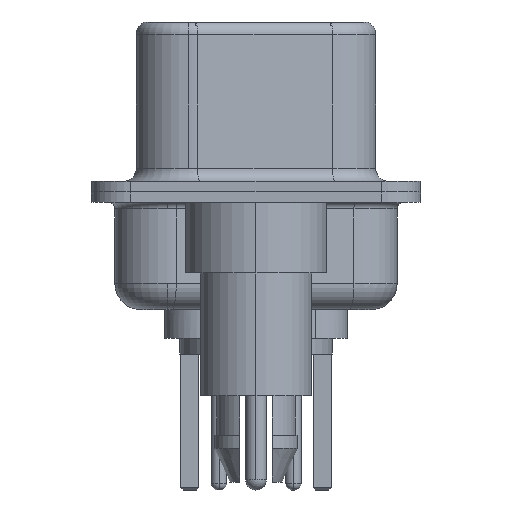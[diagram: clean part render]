
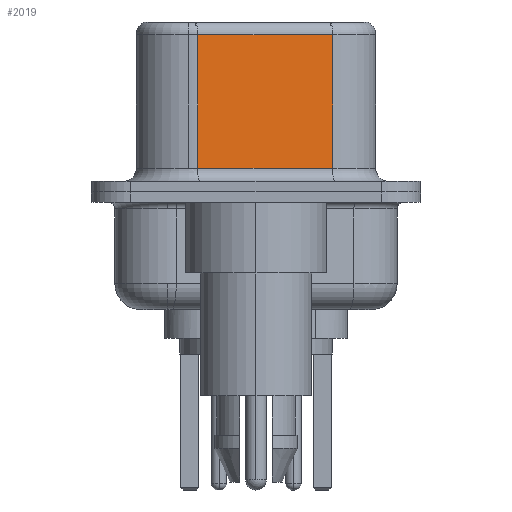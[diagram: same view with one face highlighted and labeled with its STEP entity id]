
A CAD part, left-side view. The second image highlights one B-rep face of the part: STEP entity #2019.
In plain terms, the highlighted planar face has unit normal (-0.985, -0.174, 0).
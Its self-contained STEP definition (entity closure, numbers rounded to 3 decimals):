
#1563 = LINE ( 'NONE', #5303, #13319 ) ;
#1686 = CARTESIAN_POINT ( 'NONE',  ( 4.58, -2.927, 6.02 ) ) ;
#2019 = ADVANCED_FACE ( 'NONE', ( #23854 ), #16292, .F. ) ;
#5303 = CARTESIAN_POINT ( 'NONE',  ( 3.67, 2.233, 6.52 ) ) ;
#6105 = EDGE_CURVE ( 'NONE', #13975, #22744, #17256, .T. ) ;
#6695 = AXIS2_PLACEMENT_3D ( 'NONE', #9217, #9835, #22494 ) ;
#7538 = DIRECTION ( 'NONE',  ( 0., 0., -1. ) ) ;
#7611 = DIRECTION ( 'NONE',  ( 0., 0., -1. ) ) ;
#8519 = ORIENTED_EDGE ( 'NONE', *, *, #8680, .T. ) ;
#8598 = ORIENTED_EDGE ( 'NONE', *, *, #28060, .T. ) ;
#8680 = EDGE_CURVE ( 'NONE', #28010, #22744, #13854, .T. ) ;
#9217 = CARTESIAN_POINT ( 'NONE',  ( 4.58, -2.927, 6.52 ) ) ;
#9610 = LINE ( 'NONE', #1686, #15121 ) ;
#9835 = DIRECTION ( 'NONE',  ( 0.985, 0.174, 0. ) ) ;
#10429 = VERTEX_POINT ( 'NONE', #12558 ) ;
#12558 = CARTESIAN_POINT ( 'NONE',  ( 3.67, 2.233, 6.02 ) ) ;
#13319 = VECTOR ( 'NONE', #7611, 1000. ) ;
#13854 = LINE ( 'NONE', #23013, #20037 ) ;
#13975 = VERTEX_POINT ( 'NONE', #21192 ) ;
#15121 = VECTOR ( 'NONE', #25491, 1000. ) ;
#16230 = EDGE_LOOP ( 'NONE', ( #19924, #26588, #8598, #8519 ) ) ;
#16292 = PLANE ( 'NONE',  #6695 ) ;
#17256 = LINE ( 'NONE', #22713, #29658 ) ;
#19210 = CARTESIAN_POINT ( 'NONE',  ( 3.67, 2.233, 0.9 ) ) ;
#19924 = ORIENTED_EDGE ( 'NONE', *, *, #6105, .F. ) ;
#20037 = VECTOR ( 'NONE', #25384, 1000. ) ;
#21037 = CARTESIAN_POINT ( 'NONE',  ( 4.58, -2.927, 0.9 ) ) ;
#21192 = CARTESIAN_POINT ( 'NONE',  ( 4.58, -2.927, 6.02 ) ) ;
#22494 = DIRECTION ( 'NONE',  ( -0.174, 0.985, 0. ) ) ;
#22713 = CARTESIAN_POINT ( 'NONE',  ( 4.58, -2.927, 6.52 ) ) ;
#22744 = VERTEX_POINT ( 'NONE', #21037 ) ;
#23013 = CARTESIAN_POINT ( 'NONE',  ( 4.58, -2.927, 0.9 ) ) ;
#23149 = EDGE_CURVE ( 'NONE', #13975, #10429, #9610, .T. ) ;
#23854 = FACE_OUTER_BOUND ( 'NONE', #16230, .T. ) ;
#25384 = DIRECTION ( 'NONE',  ( 0.174, -0.985, 0. ) ) ;
#25491 = DIRECTION ( 'NONE',  ( -0.174, 0.985, 0. ) ) ;
#26588 = ORIENTED_EDGE ( 'NONE', *, *, #23149, .T. ) ;
#28010 = VERTEX_POINT ( 'NONE', #19210 ) ;
#28060 = EDGE_CURVE ( 'NONE', #10429, #28010, #1563, .T. ) ;
#29658 = VECTOR ( 'NONE', #7538, 1000. ) ;
